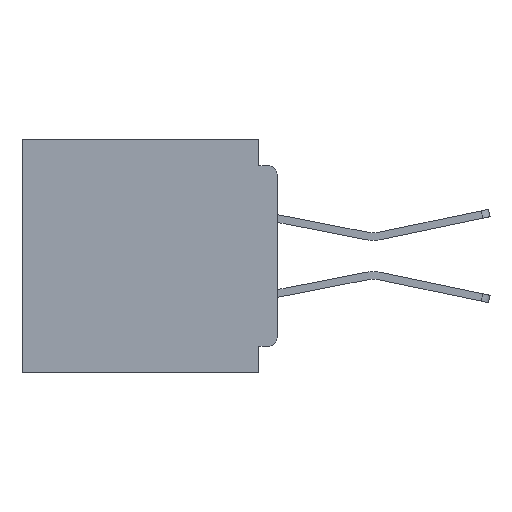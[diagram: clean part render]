
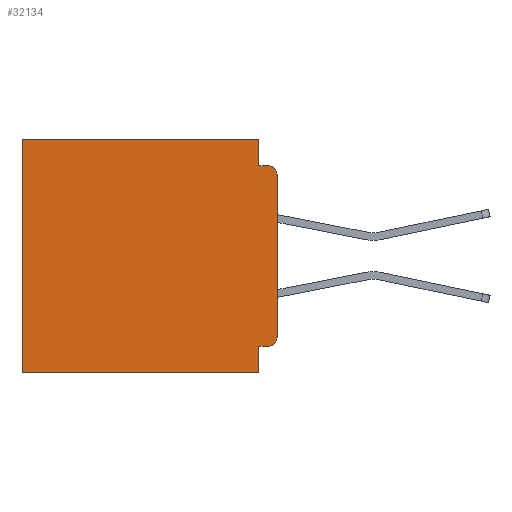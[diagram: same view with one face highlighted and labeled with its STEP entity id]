
A CAD part, left-side view. The second image highlights one B-rep face of the part: STEP entity #32134.
In plain terms, the highlighted planar face has unit normal (-1, 0, 0).
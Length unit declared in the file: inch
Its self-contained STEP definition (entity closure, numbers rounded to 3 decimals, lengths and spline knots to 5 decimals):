
#473 = VECTOR ( 'NONE', #9898, 39.37008 ) ;
#594 = LINE ( 'NONE', #14990, #15234 ) ;
#873 = EDGE_CURVE ( 'NONE', #7523, #31566, #594, .T. ) ;
#1164 = EDGE_CURVE ( 'NONE', #7060, #27590, #34130, .T. ) ;
#1272 = CARTESIAN_POINT ( 'NONE',  ( 0.3, 0.437, 0. ) ) ;
#2666 = CARTESIAN_POINT ( 'NONE',  ( 0.3, 0., -0.06 ) ) ;
#2694 = DIRECTION ( 'NONE',  ( 0., 0., -1. ) ) ;
#3562 = DIRECTION ( 'NONE',  ( -1., 0., 0. ) ) ;
#3887 = CARTESIAN_POINT ( 'NONE',  ( 0.3, 0., -0.355 ) ) ;
#4128 = LINE ( 'NONE', #9856, #32533 ) ;
#4618 = DIRECTION ( 'NONE',  ( 0., 1., 0. ) ) ;
#5337 = CARTESIAN_POINT ( 'NONE',  ( 0.3, 0., -0.4 ) ) ;
#5390 = VERTEX_POINT ( 'NONE', #13417 ) ;
#5721 = CARTESIAN_POINT ( 'NONE',  ( 0.3, 0.031, -0.4 ) ) ;
#6445 = EDGE_CURVE ( 'NONE', #27539, #7727, #6843, .T. ) ;
#6483 = ORIENTED_EDGE ( 'NONE', *, *, #873, .T. ) ;
#6710 = CIRCLE ( 'NONE', #18995, 0.015 ) ;
#6718 = CARTESIAN_POINT ( 'NONE',  ( 0.3, 0.015, -0.355 ) ) ;
#6843 = LINE ( 'NONE', #3887, #13273 ) ;
#7060 = VERTEX_POINT ( 'NONE', #34020 ) ;
#7142 = CARTESIAN_POINT ( 'NONE',  ( 0.3, 0., -0.045 ) ) ;
#7523 = VERTEX_POINT ( 'NONE', #28023 ) ;
#7727 = VERTEX_POINT ( 'NONE', #23327 ) ;
#9856 = CARTESIAN_POINT ( 'NONE',  ( 0.3, 0.437, -0.4 ) ) ;
#9898 = DIRECTION ( 'NONE',  ( 0., -1., 0. ) ) ;
#9934 = CARTESIAN_POINT ( 'NONE',  ( 0.3, 0.437, -0.4 ) ) ;
#10072 = VERTEX_POINT ( 'NONE', #2666 ) ;
#12513 = LINE ( 'NONE', #34892, #27183 ) ;
#13067 = VECTOR ( 'NONE', #4618, 39.37008 ) ;
#13204 = AXIS2_PLACEMENT_3D ( 'NONE', #16409, #19216, #2694 ) ;
#13273 = VECTOR ( 'NONE', #28711, 39.37008 ) ;
#13417 = CARTESIAN_POINT ( 'NONE',  ( 0.3, 0.015, -0.045 ) ) ;
#13428 = CARTESIAN_POINT ( 'NONE',  ( 0.3, 0.015, -0.06 ) ) ;
#13662 = AXIS2_PLACEMENT_3D ( 'NONE', #13428, #32667, #16200 ) ;
#14990 = CARTESIAN_POINT ( 'NONE',  ( 0.3, 0., 0. ) ) ;
#15101 = LINE ( 'NONE', #7142, #473 ) ;
#15234 = VECTOR ( 'NONE', #19743, 39.37008 ) ;
#15837 = ORIENTED_EDGE ( 'NONE', *, *, #1164, .F. ) ;
#16162 = EDGE_CURVE ( 'NONE', #32790, #5390, #15101, .T. ) ;
#16200 = DIRECTION ( 'NONE',  ( 0., 0., -1. ) ) ;
#16409 = CARTESIAN_POINT ( 'NONE',  ( 0.3, 0., -0.4 ) ) ;
#17395 = LINE ( 'NONE', #5721, #29449 ) ;
#17419 = CIRCLE ( 'NONE', #13662, 0.015 ) ;
#18667 = VECTOR ( 'NONE', #24675, 39.37008 ) ;
#18995 = AXIS2_PLACEMENT_3D ( 'NONE', #20075, #3562, #22849 ) ;
#19216 = DIRECTION ( 'NONE',  ( 1., 0., 0. ) ) ;
#19264 = CARTESIAN_POINT ( 'NONE',  ( 0.3, 0.031, 0. ) ) ;
#19743 = DIRECTION ( 'NONE',  ( 0., 1., 0. ) ) ;
#20075 = CARTESIAN_POINT ( 'NONE',  ( 0.3, 0.015, -0.34 ) ) ;
#20372 = ORIENTED_EDGE ( 'NONE', *, *, #31423, .T. ) ;
#20882 = VERTEX_POINT ( 'NONE', #28441 ) ;
#22849 = DIRECTION ( 'NONE',  ( 0., 0., -1. ) ) ;
#23327 = CARTESIAN_POINT ( 'NONE',  ( 0.3, 0.031, -0.355 ) ) ;
#23863 = EDGE_CURVE ( 'NONE', #10072, #5390, #17419, .T. ) ;
#24675 = DIRECTION ( 'NONE',  ( 0., 0., -1. ) ) ;
#24695 = CARTESIAN_POINT ( 'NONE',  ( 0.3, 0.031, -0.045 ) ) ;
#26642 = DIRECTION ( 'NONE',  ( 0., 0., -1. ) ) ;
#27183 = VECTOR ( 'NONE', #26642, 39.37008 ) ;
#27290 = ORIENTED_EDGE ( 'NONE', *, *, #16162, .F. ) ;
#27524 = ORIENTED_EDGE ( 'NONE', *, *, #31007, .T. ) ;
#27539 = VERTEX_POINT ( 'NONE', #6718 ) ;
#27590 = VERTEX_POINT ( 'NONE', #9934 ) ;
#28023 = CARTESIAN_POINT ( 'NONE',  ( 0.3, 0.031, 0. ) ) ;
#28441 = CARTESIAN_POINT ( 'NONE',  ( 0.3, 0., -0.34 ) ) ;
#28711 = DIRECTION ( 'NONE',  ( 0., 1., 0. ) ) ;
#29123 = DIRECTION ( 'NONE',  ( 0., 0., -1. ) ) ;
#29410 = ORIENTED_EDGE ( 'NONE', *, *, #32194, .F. ) ;
#29449 = VECTOR ( 'NONE', #33108, 39.37008 ) ;
#31007 = EDGE_CURVE ( 'NONE', #31566, #27590, #4128, .T. ) ;
#31423 = EDGE_CURVE ( 'NONE', #27539, #20882, #6710, .T. ) ;
#31545 = ORIENTED_EDGE ( 'NONE', *, *, #33343, .F. ) ;
#31566 = VERTEX_POINT ( 'NONE', #1272 ) ;
#32006 = FACE_OUTER_BOUND ( 'NONE', #35112, .T. ) ;
#32124 = ORIENTED_EDGE ( 'NONE', *, *, #34444, .F. ) ;
#32134 = ADVANCED_FACE ( 'NONE', ( #32006 ), #35623, .F. ) ;
#32194 = EDGE_CURVE ( 'NONE', #7727, #7060, #17395, .T. ) ;
#32327 = ORIENTED_EDGE ( 'NONE', *, *, #6445, .F. ) ;
#32533 = VECTOR ( 'NONE', #29123, 39.37008 ) ;
#32667 = DIRECTION ( 'NONE',  ( -1., 0., 0. ) ) ;
#32790 = VERTEX_POINT ( 'NONE', #24695 ) ;
#33108 = DIRECTION ( 'NONE',  ( 0., 0., -1. ) ) ;
#33245 = LINE ( 'NONE', #19264, #18667 ) ;
#33343 = EDGE_CURVE ( 'NONE', #7523, #32790, #33245, .T. ) ;
#33851 = ORIENTED_EDGE ( 'NONE', *, *, #23863, .T. ) ;
#34020 = CARTESIAN_POINT ( 'NONE',  ( 0.3, 0.031, -0.4 ) ) ;
#34130 = LINE ( 'NONE', #5337, #13067 ) ;
#34444 = EDGE_CURVE ( 'NONE', #10072, #20882, #12513, .T. ) ;
#34892 = CARTESIAN_POINT ( 'NONE',  ( 0.3, 0., -0.4 ) ) ;
#35112 = EDGE_LOOP ( 'NONE', ( #32124, #33851, #27290, #31545, #6483, #27524, #15837, #29410, #32327, #20372 ) ) ;
#35623 = PLANE ( 'NONE',  #13204 ) ;
